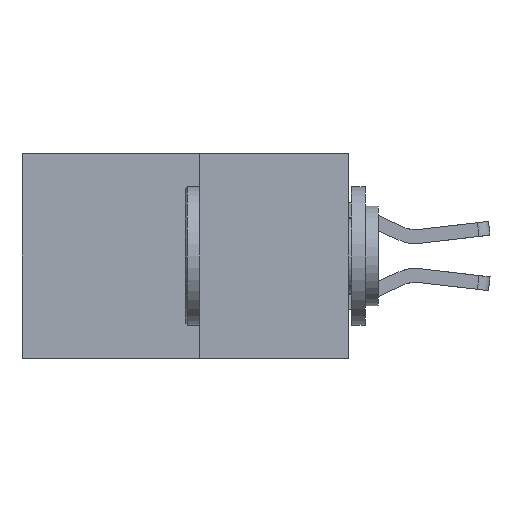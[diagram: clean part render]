
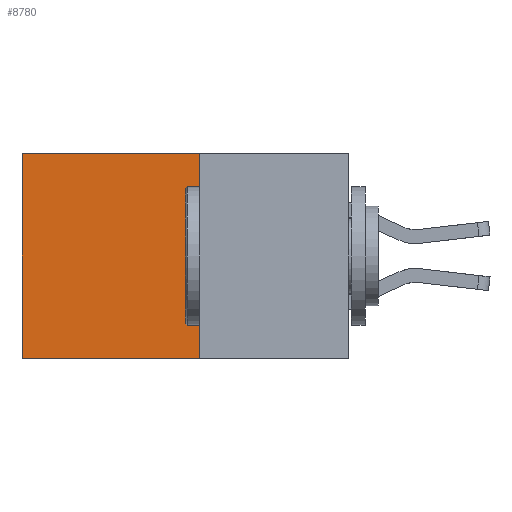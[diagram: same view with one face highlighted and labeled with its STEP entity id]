
A CAD part, left-side view. The second image highlights one B-rep face of the part: STEP entity #8780.
In plain terms, the highlighted planar face has unit normal (-1, 0, 0).
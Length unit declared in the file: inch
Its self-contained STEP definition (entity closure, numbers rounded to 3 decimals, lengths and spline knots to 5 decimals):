
#15 = EDGE_CURVE ( 'NONE', #7530, #480, #5694, .T. ) ;
#480 = VERTEX_POINT ( 'NONE', #3715 ) ;
#492 = VECTOR ( 'NONE', #3678, 39.37008 ) ;
#591 = CARTESIAN_POINT ( 'NONE',  ( 0.277, 0.59, -0.37 ) ) ;
#952 = CARTESIAN_POINT ( 'NONE',  ( 0.277, 0.27, -0.37 ) ) ;
#1002 = ORIENTED_EDGE ( 'NONE', *, *, #15, .F. ) ;
#1611 = EDGE_CURVE ( 'NONE', #5803, #5587, #2913, .T. ) ;
#1836 = VECTOR ( 'NONE', #5012, 39.37008 ) ;
#1848 = ORIENTED_EDGE ( 'NONE', *, *, #3513, .F. ) ;
#2486 = EDGE_CURVE ( 'NONE', #7530, #5803, #6732, .T. ) ;
#2508 = DIRECTION ( 'NONE',  ( 0., 0., -1. ) ) ;
#2913 = LINE ( 'NONE', #3170, #4511 ) ;
#3021 = ORIENTED_EDGE ( 'NONE', *, *, #2486, .T. ) ;
#3170 = CARTESIAN_POINT ( 'NONE',  ( 0.277, 0.59, -0.37 ) ) ;
#3399 = DIRECTION ( 'NONE',  ( 0., 0., -1. ) ) ;
#3513 = EDGE_CURVE ( 'NONE', #480, #5587, #6080, .T. ) ;
#3571 = DIRECTION ( 'NONE',  ( 0., 1., 0. ) ) ;
#3576 = EDGE_LOOP ( 'NONE', ( #4076, #1848, #1002, #3021 ) ) ;
#3678 = DIRECTION ( 'NONE',  ( 0., 0., -1. ) ) ;
#3715 = CARTESIAN_POINT ( 'NONE',  ( 0.277, 0.27, -0.37 ) ) ;
#4076 = ORIENTED_EDGE ( 'NONE', *, *, #1611, .T. ) ;
#4511 = VECTOR ( 'NONE', #3399, 39.37008 ) ;
#4908 = CARTESIAN_POINT ( 'NONE',  ( 0.277, 0.27, 0. ) ) ;
#5012 = DIRECTION ( 'NONE',  ( 0., 1., 0. ) ) ;
#5218 = CARTESIAN_POINT ( 'NONE',  ( 0.277, 0.27, -0.37 ) ) ;
#5397 = AXIS2_PLACEMENT_3D ( 'NONE', #5218, #6579, #2508 ) ;
#5539 = FACE_OUTER_BOUND ( 'NONE', #3576, .T. ) ;
#5558 = CARTESIAN_POINT ( 'NONE',  ( 0.277, 0.27, -0.37 ) ) ;
#5587 = VERTEX_POINT ( 'NONE', #591 ) ;
#5694 = LINE ( 'NONE', #5558, #492 ) ;
#5803 = VERTEX_POINT ( 'NONE', #7630 ) ;
#6080 = LINE ( 'NONE', #952, #1836 ) ;
#6579 = DIRECTION ( 'NONE',  ( 1., 0., 0. ) ) ;
#6732 = LINE ( 'NONE', #4908, #8843 ) ;
#7530 = VERTEX_POINT ( 'NONE', #8686 ) ;
#7630 = CARTESIAN_POINT ( 'NONE',  ( 0.277, 0.59, 0. ) ) ;
#8686 = CARTESIAN_POINT ( 'NONE',  ( 0.277, 0.27, 0. ) ) ;
#8695 = PLANE ( 'NONE',  #5397 ) ;
#8780 = ADVANCED_FACE ( 'NONE', ( #5539 ), #8695, .F. ) ;
#8843 = VECTOR ( 'NONE', #3571, 39.37008 ) ;
